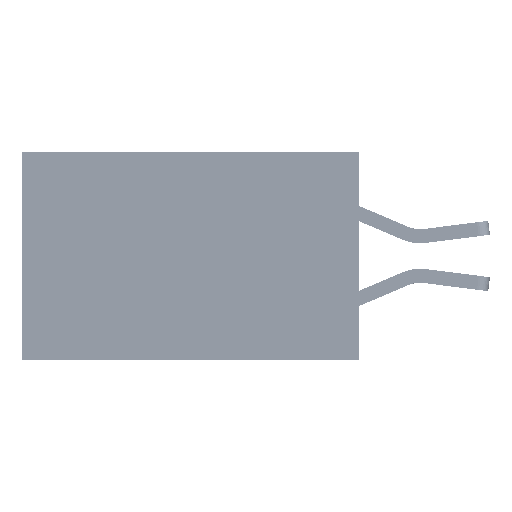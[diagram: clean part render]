
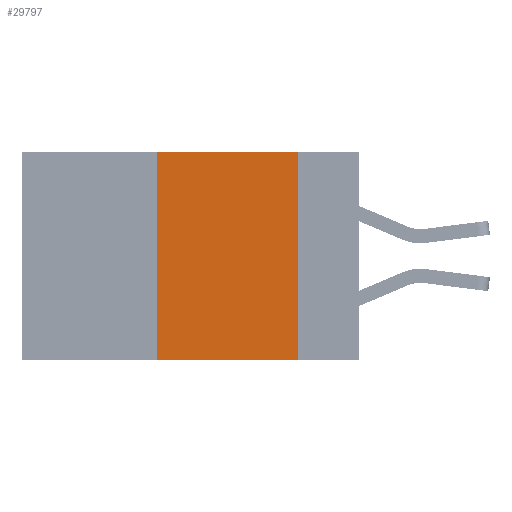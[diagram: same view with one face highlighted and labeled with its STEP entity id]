
A CAD part, left-side view. The second image highlights one B-rep face of the part: STEP entity #29797.
In plain terms, the highlighted planar face has unit normal (-1, 0, 0).
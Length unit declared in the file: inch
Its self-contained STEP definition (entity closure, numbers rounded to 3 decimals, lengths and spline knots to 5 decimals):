
#483 = LINE ( 'NONE', #21036, #22617 ) ;
#509 = LINE ( 'NONE', #28003, #7224 ) ;
#2978 = PLANE ( 'NONE',  #49827 ) ;
#5744 = LINE ( 'NONE', #12984, #32285 ) ;
#7224 = VECTOR ( 'NONE', #49348, 39.37008 ) ;
#7547 = FACE_OUTER_BOUND ( 'NONE', #36159, .T. ) ;
#8847 = VECTOR ( 'NONE', #52120, 39.37008 ) ;
#9299 = DIRECTION ( 'NONE',  ( 0., 0., -1. ) ) ;
#10070 = VERTEX_POINT ( 'NONE', #30923 ) ;
#11530 = EDGE_CURVE ( 'NONE', #20961, #24819, #509, .T. ) ;
#11656 = CARTESIAN_POINT ( 'NONE',  ( 0., 0.11, 0. ) ) ;
#12984 = CARTESIAN_POINT ( 'NONE',  ( 0., 0.6, 0. ) ) ;
#13346 = ORIENTED_EDGE ( 'NONE', *, *, #43157, .F. ) ;
#17503 = ORIENTED_EDGE ( 'NONE', *, *, #11530, .F. ) ;
#17843 = ORIENTED_EDGE ( 'NONE', *, *, #49864, .T. ) ;
#19272 = CARTESIAN_POINT ( 'NONE',  ( 0., 0.6, 0. ) ) ;
#19541 = DIRECTION ( 'NONE',  ( 1., 0., 0. ) ) ;
#19583 = LINE ( 'NONE', #39835, #8847 ) ;
#20961 = VERTEX_POINT ( 'NONE', #28064 ) ;
#21036 = CARTESIAN_POINT ( 'NONE',  ( 0., 0.11, 0. ) ) ;
#22617 = VECTOR ( 'NONE', #9299, 39.37008 ) ;
#24819 = VERTEX_POINT ( 'NONE', #33030 ) ;
#26732 = DIRECTION ( 'NONE',  ( 0., 0., -1. ) ) ;
#27501 = VERTEX_POINT ( 'NONE', #11656 ) ;
#28003 = CARTESIAN_POINT ( 'NONE',  ( 0., 0.36, 0. ) ) ;
#28064 = CARTESIAN_POINT ( 'NONE',  ( 0., 0.36, -0.37 ) ) ;
#28531 = EDGE_CURVE ( 'NONE', #27501, #10070, #483, .T. ) ;
#29797 = ADVANCED_FACE ( 'NONE', ( #7547 ), #2978, .F. ) ;
#30923 = CARTESIAN_POINT ( 'NONE',  ( 0., 0.11, -0.37 ) ) ;
#32285 = VECTOR ( 'NONE', #49770, 39.37008 ) ;
#33030 = CARTESIAN_POINT ( 'NONE',  ( 0., 0.36, 0. ) ) ;
#36159 = EDGE_LOOP ( 'NONE', ( #39255, #13346, #17503, #17843 ) ) ;
#39255 = ORIENTED_EDGE ( 'NONE', *, *, #28531, .F. ) ;
#39835 = CARTESIAN_POINT ( 'NONE',  ( 0., 0.6, -0.37 ) ) ;
#43157 = EDGE_CURVE ( 'NONE', #24819, #27501, #5744, .T. ) ;
#49348 = DIRECTION ( 'NONE',  ( 0., 0., 1. ) ) ;
#49770 = DIRECTION ( 'NONE',  ( 0., -1., 0. ) ) ;
#49827 = AXIS2_PLACEMENT_3D ( 'NONE', #19272, #19541, #26732 ) ;
#49864 = EDGE_CURVE ( 'NONE', #20961, #10070, #19583, .T. ) ;
#52120 = DIRECTION ( 'NONE',  ( 0., -1., 0. ) ) ;
